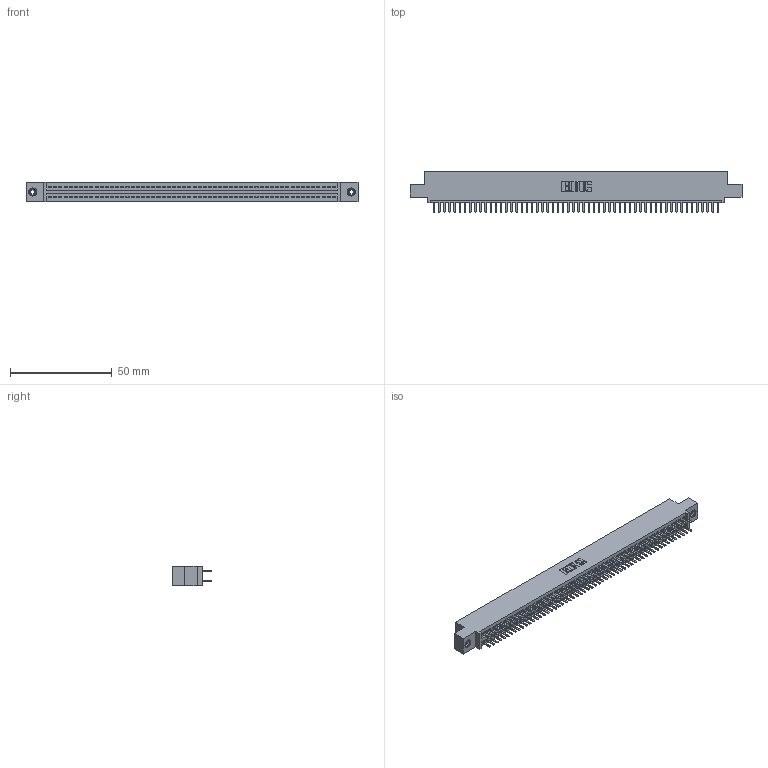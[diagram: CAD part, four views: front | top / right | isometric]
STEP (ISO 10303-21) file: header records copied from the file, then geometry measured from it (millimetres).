
FILE_DESCRIPTION (( 'STEP AP203' ), '1' );
FILE_NAME ('395-112-520-508.STEP', '2019-10-27T12:51:54', ( '' ), ( '' ), 'SwSTEP 2.0', 'SolidWorks 2016', '' );
FILE_SCHEMA (( 'CONFIG_CONTROL_DESIGN' ));
Length unit declared in the file: inch
Products named in the file (4): 345 Part_0.110 Offset - 0.156 Dia-TI; 345-292-001_345-293-120; 345-250-001_345-250-003-102; 395-112-520-508
Assembly tree (115 placements, depth 2):
  395-112-520-508
    345 Part_0.110 Offset - 0.156 Dia-TI
    345-292-001_345-293-120  x112
    345-250-001_345-250-003-102  x2
Bounding box: 163.45 x 19.68 x 9.4 mm (x, y, z)
Volume: 15878.4 mm3; surface area: 23743.7 mm2
Topology: 115 solids, 115 shells, 6238 faces, 18073 edges, 11742 vertices
Faces by surface type: plane 4036, cylinder 2186, cone 12, torus 4
Entity records: 43486 total; most frequent: CARTESIAN_POINT 7271, ORIENTED_EDGE 7186, DIRECTION 6407, EDGE_CURVE 3593, LINE 3213, VECTOR 3213, VERTEX_POINT 2388, AXIS2_PLACEMENT_3D 1597
